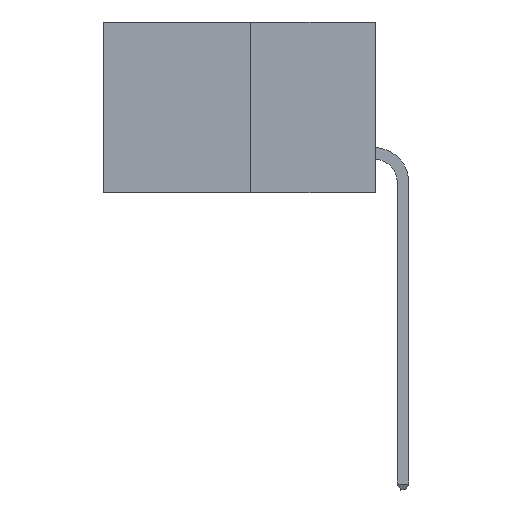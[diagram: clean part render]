
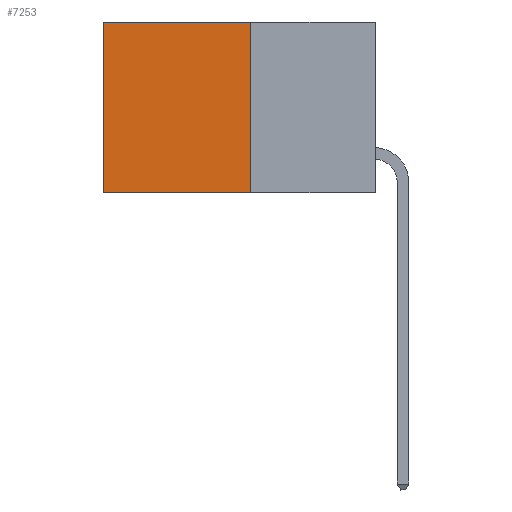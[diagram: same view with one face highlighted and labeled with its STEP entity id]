
A CAD part, left-side view. The second image highlights one B-rep face of the part: STEP entity #7253.
In plain terms, the highlighted planar face has unit normal (-1, 0, 0).
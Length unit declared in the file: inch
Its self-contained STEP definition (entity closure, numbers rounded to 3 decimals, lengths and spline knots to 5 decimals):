
#433 = CARTESIAN_POINT ( 'NONE',  ( 0.277, 0.27, 0. ) ) ;
#446 = DIRECTION ( 'NONE',  ( 0., 0., -1. ) ) ;
#786 = EDGE_CURVE ( 'NONE', #5636, #10884, #10818, .T. ) ;
#873 = DIRECTION ( 'NONE',  ( 0., 0., -1. ) ) ;
#1027 = CARTESIAN_POINT ( 'NONE',  ( 0.277, 0.27, -0.37 ) ) ;
#1413 = CARTESIAN_POINT ( 'NONE',  ( 0.277, 0.27, 0. ) ) ;
#1845 = VECTOR ( 'NONE', #9582, 39.37008 ) ;
#2765 = ORIENTED_EDGE ( 'NONE', *, *, #9576, .F. ) ;
#3125 = VECTOR ( 'NONE', #873, 39.37008 ) ;
#4024 = DIRECTION ( 'NONE',  ( 0., 1., 0. ) ) ;
#4227 = AXIS2_PLACEMENT_3D ( 'NONE', #4758, #5644, #446 ) ;
#4758 = CARTESIAN_POINT ( 'NONE',  ( 0.277, 0.27, -0.37 ) ) ;
#4843 = CARTESIAN_POINT ( 'NONE',  ( 0.277, 0.27, -0.37 ) ) ;
#4960 = EDGE_CURVE ( 'NONE', #7927, #10227, #5385, .T. ) ;
#5283 = CARTESIAN_POINT ( 'NONE',  ( 0.277, 0.59, -0.37 ) ) ;
#5385 = LINE ( 'NONE', #1027, #3125 ) ;
#5636 = VERTEX_POINT ( 'NONE', #7005 ) ;
#5644 = DIRECTION ( 'NONE',  ( 1., 0., 0. ) ) ;
#6105 = VECTOR ( 'NONE', #10116, 39.37008 ) ;
#6492 = PLANE ( 'NONE',  #4227 ) ;
#6555 = FACE_OUTER_BOUND ( 'NONE', #7819, .T. ) ;
#7005 = CARTESIAN_POINT ( 'NONE',  ( 0.277, 0.59, 0. ) ) ;
#7253 = ADVANCED_FACE ( 'NONE', ( #6555 ), #6492, .F. ) ;
#7819 = EDGE_LOOP ( 'NONE', ( #10672, #2765, #7888, #9084 ) ) ;
#7888 = ORIENTED_EDGE ( 'NONE', *, *, #4960, .F. ) ;
#7927 = VERTEX_POINT ( 'NONE', #433 ) ;
#8157 = VECTOR ( 'NONE', #4024, 39.37008 ) ;
#8433 = LINE ( 'NONE', #1413, #8157 ) ;
#8471 = LINE ( 'NONE', #4843, #6105 ) ;
#9024 = CARTESIAN_POINT ( 'NONE',  ( 0.277, 0.59, -0.37 ) ) ;
#9084 = ORIENTED_EDGE ( 'NONE', *, *, #11240, .T. ) ;
#9576 = EDGE_CURVE ( 'NONE', #10227, #10884, #8471, .T. ) ;
#9582 = DIRECTION ( 'NONE',  ( 0., 0., -1. ) ) ;
#10116 = DIRECTION ( 'NONE',  ( 0., 1., 0. ) ) ;
#10227 = VERTEX_POINT ( 'NONE', #10413 ) ;
#10413 = CARTESIAN_POINT ( 'NONE',  ( 0.277, 0.27, -0.37 ) ) ;
#10672 = ORIENTED_EDGE ( 'NONE', *, *, #786, .T. ) ;
#10818 = LINE ( 'NONE', #9024, #1845 ) ;
#10884 = VERTEX_POINT ( 'NONE', #5283 ) ;
#11240 = EDGE_CURVE ( 'NONE', #7927, #5636, #8433, .T. ) ;
